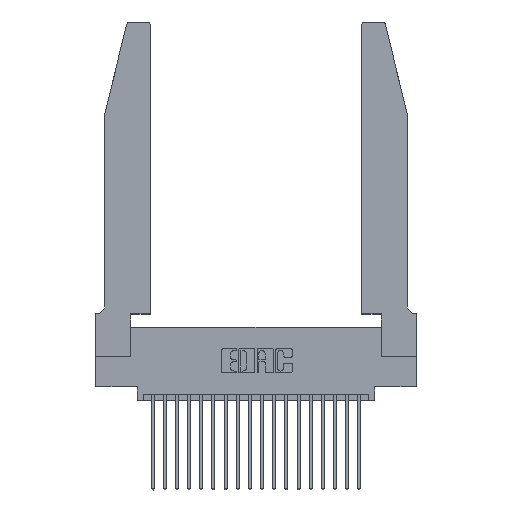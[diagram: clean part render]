
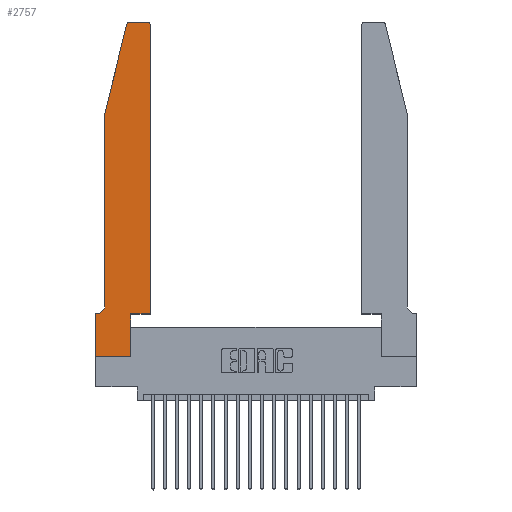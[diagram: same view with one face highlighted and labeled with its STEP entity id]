
A CAD part, top view. The second image highlights one B-rep face of the part: STEP entity #2757.
In plain terms, the highlighted planar face has unit normal (0, 0, 1).
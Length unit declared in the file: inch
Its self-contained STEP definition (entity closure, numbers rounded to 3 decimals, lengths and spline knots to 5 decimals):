
#314 = ORIENTED_EDGE ( 'NONE', *, *, #17338, .T. ) ;
#386 = DIRECTION ( 'NONE',  ( 0., 1., 0. ) ) ;
#555 = CARTESIAN_POINT ( 'NONE',  ( 0.284, 2.72, 0.37 ) ) ;
#585 = DIRECTION ( 'NONE',  ( -1., 0., 0. ) ) ;
#701 = CARTESIAN_POINT ( 'NONE',  ( 0.2605, 2.75, 0.37 ) ) ;
#1007 = ORIENTED_EDGE ( 'NONE', *, *, #15249, .T. ) ;
#1705 = ORIENTED_EDGE ( 'NONE', *, *, #14728, .T. ) ;
#1760 = CARTESIAN_POINT ( 'NONE',  ( 0.0755, 0.35, 0.37 ) ) ;
#1991 = LINE ( 'NONE', #15972, #9248 ) ;
#2147 = VECTOR ( 'NONE', #19876, 39.37008 ) ;
#2559 = VERTEX_POINT ( 'NONE', #15017 ) ;
#2757 = ADVANCED_FACE ( 'NONE', ( #3332 ), #18354, .T. ) ;
#2974 = CARTESIAN_POINT ( 'NONE',  ( 0.0755, 2., 0.37 ) ) ;
#3191 = ORIENTED_EDGE ( 'NONE', *, *, #9283, .T. ) ;
#3201 = CARTESIAN_POINT ( 'NONE',  ( 0., 0.35, 0.37 ) ) ;
#3332 = FACE_OUTER_BOUND ( 'NONE', #17610, .T. ) ;
#3371 = AXIS2_PLACEMENT_3D ( 'NONE', #555, #9222, #21091 ) ;
#3452 = EDGE_CURVE ( 'NONE', #2559, #18461, #20270, .T. ) ;
#3654 = VERTEX_POINT ( 'NONE', #21877 ) ;
#3838 = DIRECTION ( 'NONE',  ( 0., 0., -1. ) ) ;
#4067 = DIRECTION ( 'NONE',  ( 0., -1., 0. ) ) ;
#4160 = VECTOR ( 'NONE', #9681, 39.37008 ) ;
#4182 = DIRECTION ( 'NONE',  ( -0.239, -0.971, 0. ) ) ;
#4199 = LINE ( 'NONE', #1760, #13401 ) ;
#4474 = CARTESIAN_POINT ( 'NONE',  ( 0., 0., 0.37 ) ) ;
#4560 = LINE ( 'NONE', #701, #2147 ) ;
#4589 = DIRECTION ( 'NONE',  ( 1., 0., 0. ) ) ;
#5206 = ORIENTED_EDGE ( 'NONE', *, *, #14558, .T. ) ;
#5229 = CARTESIAN_POINT ( 'NONE',  ( 0.2865, 0.35, 0.37 ) ) ;
#5559 = LINE ( 'NONE', #6323, #12555 ) ;
#5829 = CARTESIAN_POINT ( 'NONE',  ( 0.284, 2.75, 0.37 ) ) ;
#6161 = ORIENTED_EDGE ( 'NONE', *, *, #19507, .T. ) ;
#6305 = CARTESIAN_POINT ( 'NONE',  ( 0.4505, 0.35, 0.37 ) ) ;
#6323 = CARTESIAN_POINT ( 'NONE',  ( 0., 0., 0.37 ) ) ;
#6557 = VERTEX_POINT ( 'NONE', #3201 ) ;
#6719 = ORIENTED_EDGE ( 'NONE', *, *, #11290, .T. ) ;
#7116 = VECTOR ( 'NONE', #10361, 39.37008 ) ;
#7278 = EDGE_CURVE ( 'NONE', #13264, #2559, #5559, .T. ) ;
#7340 = EDGE_CURVE ( 'NONE', #18585, #10343, #14411, .T. ) ;
#7794 = CIRCLE ( 'NONE', #3371, 0.03 ) ;
#7893 = AXIS2_PLACEMENT_3D ( 'NONE', #19799, #3838, #16101 ) ;
#7905 = DIRECTION ( 'NONE',  ( 0., 0., 1. ) ) ;
#8066 = DIRECTION ( 'NONE',  ( 1., 0., 0. ) ) ;
#8730 = VECTOR ( 'NONE', #16047, 39.37008 ) ;
#8755 = ORIENTED_EDGE ( 'NONE', *, *, #17310, .T. ) ;
#8776 = VERTEX_POINT ( 'NONE', #19036 ) ;
#9222 = DIRECTION ( 'NONE',  ( 0., 0., 1. ) ) ;
#9248 = VECTOR ( 'NONE', #386, 39.37008 ) ;
#9283 = EDGE_CURVE ( 'NONE', #14771, #20900, #14868, .T. ) ;
#9449 = ORIENTED_EDGE ( 'NONE', *, *, #17402, .T. ) ;
#9681 = DIRECTION ( 'NONE',  ( 0., -1., 0. ) ) ;
#9731 = CARTESIAN_POINT ( 'NONE',  ( 0.4205, 2.75, 0.37 ) ) ;
#10268 = CARTESIAN_POINT ( 'NONE',  ( 0., 0., 0.37 ) ) ;
#10343 = VERTEX_POINT ( 'NONE', #2974 ) ;
#10361 = DIRECTION ( 'NONE',  ( 0., 1., 0. ) ) ;
#10413 = CARTESIAN_POINT ( 'NONE',  ( 0.0755, 2., 0.37 ) ) ;
#10863 = LINE ( 'NONE', #12520, #8730 ) ;
#11000 = CARTESIAN_POINT ( 'NONE',  ( 0.0755, 2., 0.37 ) ) ;
#11290 = EDGE_CURVE ( 'NONE', #20900, #16823, #4560, .T. ) ;
#11509 = CARTESIAN_POINT ( 'NONE',  ( 0.4205, 2.72, 0.37 ) ) ;
#12520 = CARTESIAN_POINT ( 'NONE',  ( 0.4505, 0.35, 0.37 ) ) ;
#12522 = VERTEX_POINT ( 'NONE', #6305 ) ;
#12555 = VECTOR ( 'NONE', #8066, 39.37008 ) ;
#13237 = DIRECTION ( 'NONE',  ( 1., 0., 0. ) ) ;
#13264 = VERTEX_POINT ( 'NONE', #10268 ) ;
#13313 = ORIENTED_EDGE ( 'NONE', *, *, #7340, .T. ) ;
#13401 = VECTOR ( 'NONE', #585, 39.37008 ) ;
#13608 = ORIENTED_EDGE ( 'NONE', *, *, #7278, .T. ) ;
#13995 = AXIS2_PLACEMENT_3D ( 'NONE', #11509, #21703, #13237 ) ;
#14411 = LINE ( 'NONE', #10413, #15793 ) ;
#14558 = EDGE_CURVE ( 'NONE', #3654, #6557, #4199, .T. ) ;
#14728 = EDGE_CURVE ( 'NONE', #8776, #3654, #19282, .T. ) ;
#14771 = VERTEX_POINT ( 'NONE', #18440 ) ;
#14868 = CIRCLE ( 'NONE', #13995, 0.03 ) ;
#15017 = CARTESIAN_POINT ( 'NONE',  ( 0.2865, 0., 0.37 ) ) ;
#15249 = EDGE_CURVE ( 'NONE', #6557, #13264, #16867, .T. ) ;
#15450 = VECTOR ( 'NONE', #4067, 39.37008 ) ;
#15793 = VECTOR ( 'NONE', #4182, 39.37008 ) ;
#15972 = CARTESIAN_POINT ( 'NONE',  ( 0.4505, 0.35, 0.37 ) ) ;
#16047 = DIRECTION ( 'NONE',  ( 1., 0., 0. ) ) ;
#16101 = DIRECTION ( 'NONE',  ( -1., 0., 0. ) ) ;
#16493 = CARTESIAN_POINT ( 'NONE',  ( 0., 0.35, 0.37 ) ) ;
#16823 = VERTEX_POINT ( 'NONE', #5829 ) ;
#16867 = LINE ( 'NONE', #4474, #4160 ) ;
#17189 = CARTESIAN_POINT ( 'NONE',  ( 0.25487, 2.72718, 0.37 ) ) ;
#17310 = EDGE_CURVE ( 'NONE', #12522, #14771, #1991, .T. ) ;
#17338 = EDGE_CURVE ( 'NONE', #18461, #12522, #10863, .T. ) ;
#17402 = EDGE_CURVE ( 'NONE', #10343, #8776, #20249, .T. ) ;
#17610 = EDGE_LOOP ( 'NONE', ( #6719, #6161, #13313, #9449, #1705, #5206, #1007, #13608, #18549, #314, #8755, #3191 ) ) ;
#18354 = PLANE ( 'NONE',  #21796 ) ;
#18440 = CARTESIAN_POINT ( 'NONE',  ( 0.4505, 2.72, 0.37 ) ) ;
#18461 = VERTEX_POINT ( 'NONE', #20398 ) ;
#18549 = ORIENTED_EDGE ( 'NONE', *, *, #3452, .T. ) ;
#18585 = VERTEX_POINT ( 'NONE', #17189 ) ;
#19036 = CARTESIAN_POINT ( 'NONE',  ( 0.0755, 0.42, 0.37 ) ) ;
#19282 = CIRCLE ( 'NONE', #7893, 0.07 ) ;
#19507 = EDGE_CURVE ( 'NONE', #16823, #18585, #7794, .T. ) ;
#19799 = CARTESIAN_POINT ( 'NONE',  ( 0.0055, 0.42, 0.37 ) ) ;
#19876 = DIRECTION ( 'NONE',  ( -1., 0., 0. ) ) ;
#20249 = LINE ( 'NONE', #11000, #15450 ) ;
#20270 = LINE ( 'NONE', #5229, #7116 ) ;
#20398 = CARTESIAN_POINT ( 'NONE',  ( 0.2865, 0.35, 0.37 ) ) ;
#20900 = VERTEX_POINT ( 'NONE', #9731 ) ;
#21091 = DIRECTION ( 'NONE',  ( 1., 0., 0. ) ) ;
#21703 = DIRECTION ( 'NONE',  ( 0., 0., 1. ) ) ;
#21796 = AXIS2_PLACEMENT_3D ( 'NONE', #16493, #7905, #4589 ) ;
#21877 = CARTESIAN_POINT ( 'NONE',  ( 0.0055, 0.35, 0.37 ) ) ;
